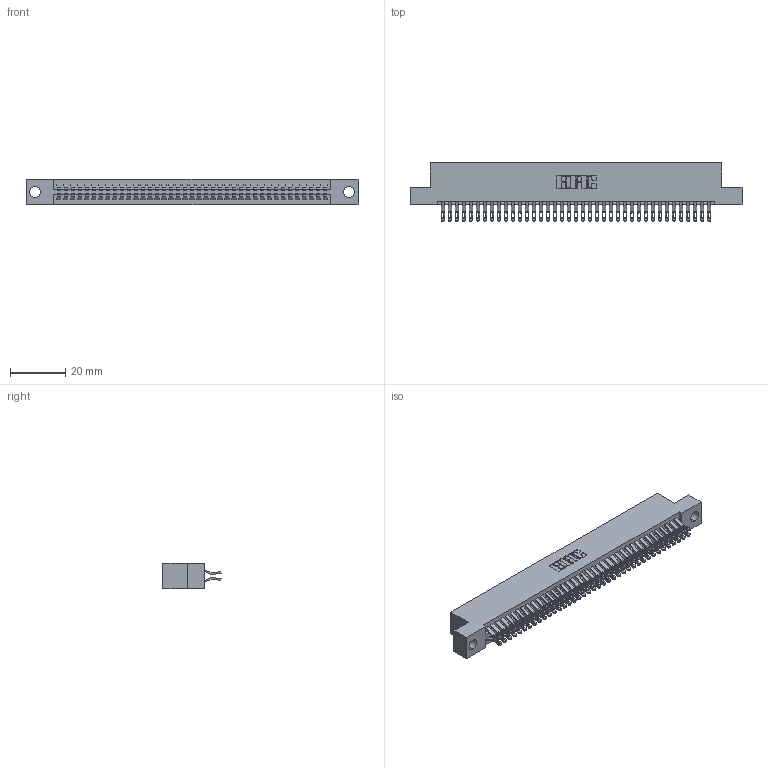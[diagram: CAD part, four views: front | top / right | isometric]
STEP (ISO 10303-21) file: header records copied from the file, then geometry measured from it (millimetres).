
FILE_DESCRIPTION (( 'STEP AP203' ), '1' );
FILE_NAME ('345-078-555-204.STEP', '2021-05-20T10:53:03', ( '' ), ( '' ), 'SwSTEP 2.0', 'SolidWorks 2020', '' );
FILE_SCHEMA (( 'CONFIG_CONTROL_DESIGN' ));
Length unit declared in the file: inch
Products named in the file (3): 345 Part_Flush Mounting Lugs - 0.156 Dia-TI; 345-078-555-204; 345-292-001_555 Tail
Assembly tree (79 placements, depth 2):
  345-078-555-204
    345 Part_Flush Mounting Lugs - 0.156 Dia-TI
    345-292-001_555 Tail  x78
Bounding box: 120.27 x 21.13 x 9.4 mm (x, y, z)
Volume: 11775.5 mm3; surface area: 17986.6 mm2
Topology: 79 solids, 79 shells, 4508 faces, 14183 edges, 9454 vertices
Faces by surface type: plane 2512, cylinder 1996
Entity records: 31749 total; most frequent: CARTESIAN_POINT 5364, ORIENTED_EDGE 5266, DIRECTION 4701, EDGE_CURVE 2633, LINE 2325, VECTOR 2325, VERTEX_POINT 1754, AXIS2_PLACEMENT_3D 1188
